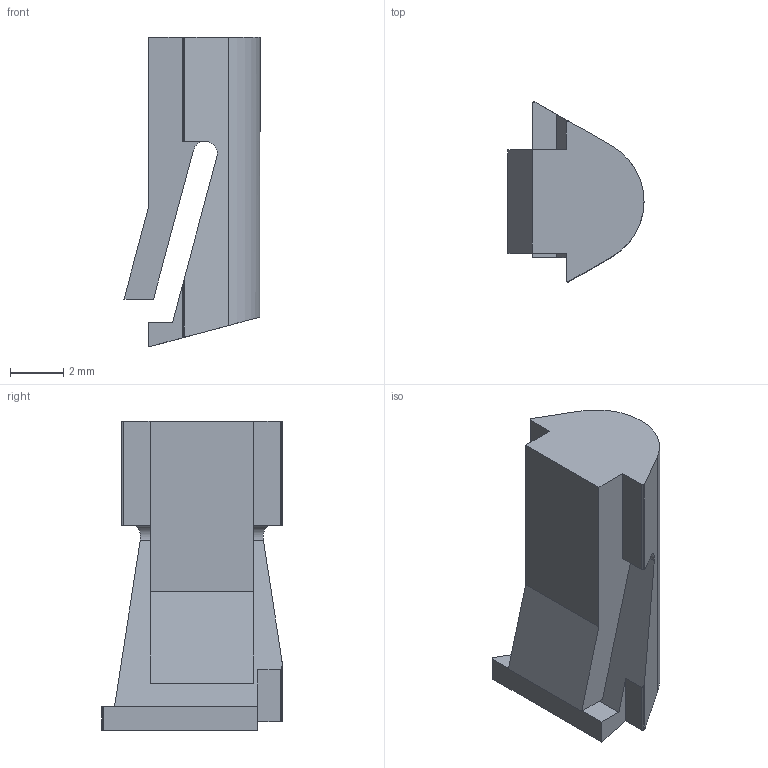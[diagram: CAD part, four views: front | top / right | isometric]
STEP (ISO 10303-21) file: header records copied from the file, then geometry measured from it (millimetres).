
FILE_DESCRIPTION (( 'STEP AP214' ), '1' );
FILE_NAME ('Magazine Catch Stop.step', '2014-07-30T19:46:06', ( 'WarFairy' ), ( '' ), 'SwSTEP 2.0', 'SolidWorks 2013', '' );
FILE_SCHEMA (( 'AUTOMOTIVE_DESIGN' ));
Length unit declared in the file: millimetre
Products named in the file (1): Magazine Catch Stop
Bounding box: 5.09 x 6.75 x 11.6 mm (x, y, z)
Volume: 166.9 mm3; surface area: 279.1 mm2
Topology: 1 solids, 1 shells, 29 faces, 81 edges, 54 vertices
Faces by surface type: plane 19, cylinder 10
Entity records: 962 total; most frequent: CARTESIAN_POINT 192, ORIENTED_EDGE 162, DIRECTION 145, EDGE_CURVE 81, LINE 59, VECTOR 59, VERTEX_POINT 54, AXIS2_PLACEMENT_3D 43
